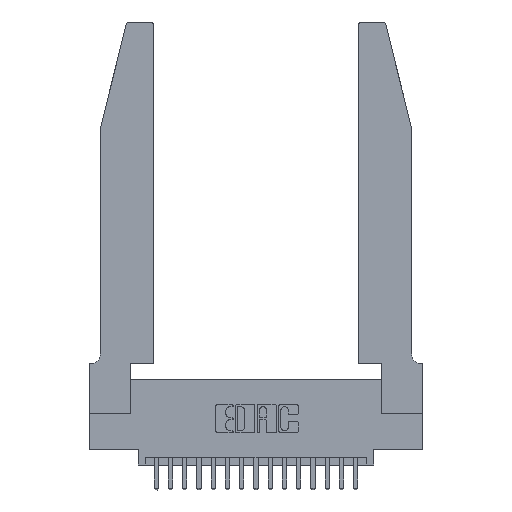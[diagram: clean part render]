
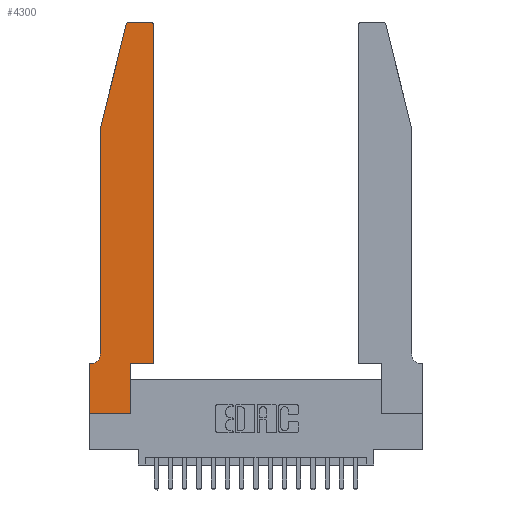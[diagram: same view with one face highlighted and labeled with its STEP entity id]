
A CAD part, top view. The second image highlights one B-rep face of the part: STEP entity #4300.
In plain terms, the highlighted planar face has unit normal (0, 0, 1).
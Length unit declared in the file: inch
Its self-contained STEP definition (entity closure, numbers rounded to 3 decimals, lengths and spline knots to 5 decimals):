
#60 = CARTESIAN_POINT ( 'NONE',  ( 0.25487, 2.72718, 0.37 ) ) ;
#187 = EDGE_CURVE ( 'NONE', #6645, #9587, #2813, .T. ) ;
#232 = FACE_OUTER_BOUND ( 'NONE', #19354, .T. ) ;
#259 = DIRECTION ( 'NONE',  ( -1., 0., 0. ) ) ;
#408 = CARTESIAN_POINT ( 'NONE',  ( 0.284, 2.72, 0.37 ) ) ;
#804 = EDGE_CURVE ( 'NONE', #2987, #808, #7706, .T. ) ;
#808 = VERTEX_POINT ( 'NONE', #18142 ) ;
#1245 = ORIENTED_EDGE ( 'NONE', *, *, #20126, .T. ) ;
#1508 = VERTEX_POINT ( 'NONE', #20386 ) ;
#1800 = ORIENTED_EDGE ( 'NONE', *, *, #13937, .T. ) ;
#1816 = CARTESIAN_POINT ( 'NONE',  ( 0.4505, 0.35, 0.37 ) ) ;
#1872 = EDGE_CURVE ( 'NONE', #808, #12128, #10730, .T. ) ;
#2002 = DIRECTION ( 'NONE',  ( 0., -1., 0. ) ) ;
#2275 = AXIS2_PLACEMENT_3D ( 'NONE', #10898, #6255, #9214 ) ;
#2414 = PLANE ( 'NONE',  #7752 ) ;
#2586 = DIRECTION ( 'NONE',  ( 0., 0., -1. ) ) ;
#2813 = CIRCLE ( 'NONE', #20256, 0.03 ) ;
#2987 = VERTEX_POINT ( 'NONE', #9617 ) ;
#3338 = EDGE_CURVE ( 'NONE', #13017, #6645, #17780, .T. ) ;
#3534 = DIRECTION ( 'NONE',  ( 0., 0., 1. ) ) ;
#3625 = LINE ( 'NONE', #3745, #12982 ) ;
#3745 = CARTESIAN_POINT ( 'NONE',  ( 0., 0., 0.37 ) ) ;
#3750 = AXIS2_PLACEMENT_3D ( 'NONE', #15125, #2586, #14156 ) ;
#3760 = CIRCLE ( 'NONE', #2275, 0.03 ) ;
#4135 = VECTOR ( 'NONE', #15776, 39.37008 ) ;
#4278 = CARTESIAN_POINT ( 'NONE',  ( 0.2865, 0.35, 0.37 ) ) ;
#4300 = ADVANCED_FACE ( 'NONE', ( #232 ), #2414, .T. ) ;
#4324 = LINE ( 'NONE', #5543, #14663 ) ;
#4794 = CARTESIAN_POINT ( 'NONE',  ( 0.4505, 0.35, 0.37 ) ) ;
#4832 = CARTESIAN_POINT ( 'NONE',  ( 0.4205, 2.75, 0.37 ) ) ;
#5184 = ORIENTED_EDGE ( 'NONE', *, *, #804, .T. ) ;
#5216 = ORIENTED_EDGE ( 'NONE', *, *, #3338, .T. ) ;
#5543 = CARTESIAN_POINT ( 'NONE',  ( 0., 0., 0.37 ) ) ;
#5671 = ORIENTED_EDGE ( 'NONE', *, *, #11070, .T. ) ;
#6255 = DIRECTION ( 'NONE',  ( 0., 0., 1. ) ) ;
#6268 = EDGE_CURVE ( 'NONE', #16908, #9075, #14480, .T. ) ;
#6301 = EDGE_CURVE ( 'NONE', #12555, #2987, #15673, .T. ) ;
#6645 = VERTEX_POINT ( 'NONE', #12117 ) ;
#6759 = DIRECTION ( 'NONE',  ( 1., 0., 0. ) ) ;
#7374 = CARTESIAN_POINT ( 'NONE',  ( 0.4505, 2.72, 0.37 ) ) ;
#7686 = DIRECTION ( 'NONE',  ( -1., 0., 0. ) ) ;
#7706 = CIRCLE ( 'NONE', #3750, 0.07 ) ;
#7752 = AXIS2_PLACEMENT_3D ( 'NONE', #16315, #17904, #17973 ) ;
#8175 = CARTESIAN_POINT ( 'NONE',  ( 0.4505, 0.35, 0.37 ) ) ;
#8534 = ORIENTED_EDGE ( 'NONE', *, *, #9248, .T. ) ;
#8776 = LINE ( 'NONE', #8175, #10800 ) ;
#9075 = VERTEX_POINT ( 'NONE', #1816 ) ;
#9214 = DIRECTION ( 'NONE',  ( 1., 0., 0. ) ) ;
#9248 = EDGE_CURVE ( 'NONE', #11731, #1508, #3625, .T. ) ;
#9308 = ORIENTED_EDGE ( 'NONE', *, *, #12972, .T. ) ;
#9570 = ORIENTED_EDGE ( 'NONE', *, *, #1872, .T. ) ;
#9587 = VERTEX_POINT ( 'NONE', #60 ) ;
#9617 = CARTESIAN_POINT ( 'NONE',  ( 0.0755, 0.42, 0.37 ) ) ;
#9746 = CARTESIAN_POINT ( 'NONE',  ( 0.0755, 2., 0.37 ) ) ;
#9999 = CARTESIAN_POINT ( 'NONE',  ( 0.0755, 2., 0.37 ) ) ;
#10730 = LINE ( 'NONE', #16097, #18332 ) ;
#10800 = VECTOR ( 'NONE', #19323, 39.37008 ) ;
#10898 = CARTESIAN_POINT ( 'NONE',  ( 0.4205, 2.72, 0.37 ) ) ;
#11070 = EDGE_CURVE ( 'NONE', #9587, #12555, #14179, .T. ) ;
#11731 = VERTEX_POINT ( 'NONE', #15569 ) ;
#11963 = VECTOR ( 'NONE', #17674, 39.37008 ) ;
#12046 = CARTESIAN_POINT ( 'NONE',  ( 0., 0.35, 0.37 ) ) ;
#12117 = CARTESIAN_POINT ( 'NONE',  ( 0.284, 2.75, 0.37 ) ) ;
#12128 = VERTEX_POINT ( 'NONE', #12046 ) ;
#12189 = ORIENTED_EDGE ( 'NONE', *, *, #6301, .T. ) ;
#12501 = VECTOR ( 'NONE', #2002, 39.37008 ) ;
#12555 = VERTEX_POINT ( 'NONE', #19604 ) ;
#12603 = ORIENTED_EDGE ( 'NONE', *, *, #19235, .T. ) ;
#12972 = EDGE_CURVE ( 'NONE', #20209, #13017, #3760, .T. ) ;
#12982 = VECTOR ( 'NONE', #16050, 39.37008 ) ;
#13017 = VERTEX_POINT ( 'NONE', #4832 ) ;
#13583 = VECTOR ( 'NONE', #7686, 39.37008 ) ;
#13656 = CARTESIAN_POINT ( 'NONE',  ( 0.2865, 0.35, 0.37 ) ) ;
#13937 = EDGE_CURVE ( 'NONE', #1508, #16908, #17263, .T. ) ;
#13953 = CARTESIAN_POINT ( 'NONE',  ( 0.2605, 2.75, 0.37 ) ) ;
#13989 = ORIENTED_EDGE ( 'NONE', *, *, #187, .T. ) ;
#14156 = DIRECTION ( 'NONE',  ( -1., 0., 0. ) ) ;
#14179 = LINE ( 'NONE', #9746, #11963 ) ;
#14480 = LINE ( 'NONE', #4794, #4135 ) ;
#14554 = VECTOR ( 'NONE', #15035, 39.37008 ) ;
#14663 = VECTOR ( 'NONE', #14756, 39.37008 ) ;
#14756 = DIRECTION ( 'NONE',  ( 0., -1., 0. ) ) ;
#15035 = DIRECTION ( 'NONE',  ( 0., 1., 0. ) ) ;
#15125 = CARTESIAN_POINT ( 'NONE',  ( 0.0055, 0.42, 0.37 ) ) ;
#15569 = CARTESIAN_POINT ( 'NONE',  ( 0., 0., 0.37 ) ) ;
#15616 = ORIENTED_EDGE ( 'NONE', *, *, #6268, .T. ) ;
#15673 = LINE ( 'NONE', #9999, #12501 ) ;
#15776 = DIRECTION ( 'NONE',  ( 1., 0., 0. ) ) ;
#16050 = DIRECTION ( 'NONE',  ( 1., 0., 0. ) ) ;
#16097 = CARTESIAN_POINT ( 'NONE',  ( 0.0755, 0.35, 0.37 ) ) ;
#16315 = CARTESIAN_POINT ( 'NONE',  ( 0., 0.35, 0.37 ) ) ;
#16908 = VERTEX_POINT ( 'NONE', #4278 ) ;
#17263 = LINE ( 'NONE', #13656, #14554 ) ;
#17674 = DIRECTION ( 'NONE',  ( -0.239, -0.971, 0. ) ) ;
#17780 = LINE ( 'NONE', #13953, #13583 ) ;
#17904 = DIRECTION ( 'NONE',  ( 0., 0., 1. ) ) ;
#17973 = DIRECTION ( 'NONE',  ( 1., 0., 0. ) ) ;
#18142 = CARTESIAN_POINT ( 'NONE',  ( 0.0055, 0.35, 0.37 ) ) ;
#18332 = VECTOR ( 'NONE', #259, 39.37008 ) ;
#19235 = EDGE_CURVE ( 'NONE', #9075, #20209, #8776, .T. ) ;
#19323 = DIRECTION ( 'NONE',  ( 0., 1., 0. ) ) ;
#19354 = EDGE_LOOP ( 'NONE', ( #5216, #13989, #5671, #12189, #5184, #9570, #1245, #8534, #1800, #15616, #12603, #9308 ) ) ;
#19604 = CARTESIAN_POINT ( 'NONE',  ( 0.0755, 2., 0.37 ) ) ;
#20126 = EDGE_CURVE ( 'NONE', #12128, #11731, #4324, .T. ) ;
#20209 = VERTEX_POINT ( 'NONE', #7374 ) ;
#20256 = AXIS2_PLACEMENT_3D ( 'NONE', #408, #3534, #6759 ) ;
#20386 = CARTESIAN_POINT ( 'NONE',  ( 0.2865, 0., 0.37 ) ) ;
